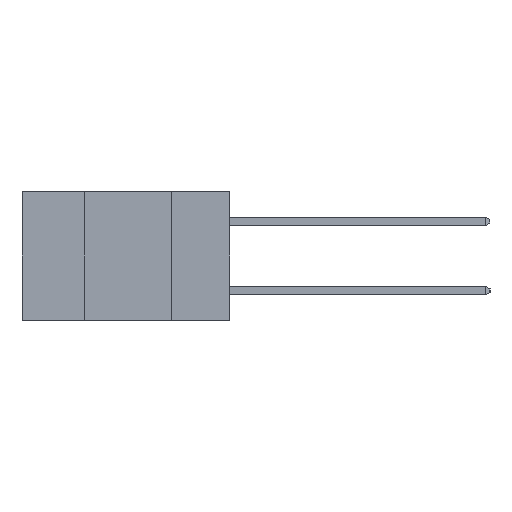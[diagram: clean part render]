
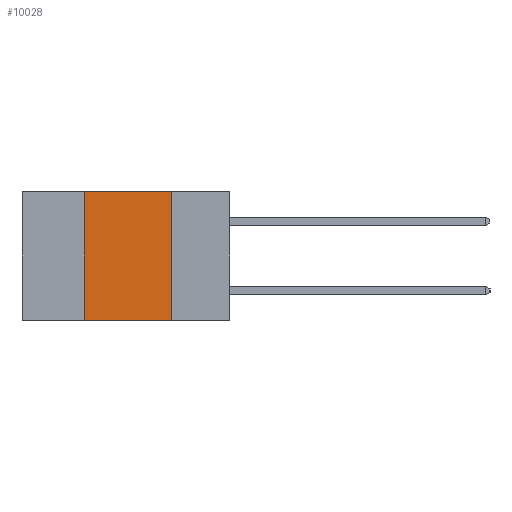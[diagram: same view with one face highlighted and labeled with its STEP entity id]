
A CAD part, left-side view. The second image highlights one B-rep face of the part: STEP entity #10028.
In plain terms, the highlighted planar face has unit normal (-1, 0, 0).
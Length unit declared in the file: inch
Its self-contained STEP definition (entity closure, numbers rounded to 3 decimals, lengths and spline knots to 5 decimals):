
#29 = DIRECTION ( 'NONE',  ( 0., 0., 1. ) ) ;
#115 = LINE ( 'NONE', #14976, #8903 ) ;
#502 = CARTESIAN_POINT ( 'NONE',  ( 0., 0.17, -0.37 ) ) ;
#624 = ORIENTED_EDGE ( 'NONE', *, *, #6920, .T. ) ;
#657 = CARTESIAN_POINT ( 'NONE',  ( 0., 0.42, 0. ) ) ;
#780 = VERTEX_POINT ( 'NONE', #4286 ) ;
#1017 = EDGE_CURVE ( 'NONE', #4652, #780, #13399, .T. ) ;
#2621 = ORIENTED_EDGE ( 'NONE', *, *, #6716, .F. ) ;
#3470 = AXIS2_PLACEMENT_3D ( 'NONE', #11093, #11650, #11632 ) ;
#3851 = EDGE_LOOP ( 'NONE', ( #14650, #2621, #12785, #624 ) ) ;
#4035 = VECTOR ( 'NONE', #13903, 39.37008 ) ;
#4286 = CARTESIAN_POINT ( 'NONE',  ( 0., 0.17, -0.37 ) ) ;
#4652 = VERTEX_POINT ( 'NONE', #10994 ) ;
#4947 = FACE_OUTER_BOUND ( 'NONE', #3851, .T. ) ;
#6237 = LINE ( 'NONE', #13095, #14942 ) ;
#6617 = VERTEX_POINT ( 'NONE', #11918 ) ;
#6716 = EDGE_CURVE ( 'NONE', #13070, #4652, #6237, .T. ) ;
#6920 = EDGE_CURVE ( 'NONE', #6617, #780, #12240, .T. ) ;
#6927 = DIRECTION ( 'NONE',  ( 0., -1., 0. ) ) ;
#7450 = CARTESIAN_POINT ( 'NONE',  ( 0., 0.6, -0.37 ) ) ;
#8903 = VECTOR ( 'NONE', #29, 39.37008 ) ;
#9192 = VECTOR ( 'NONE', #6927, 39.37008 ) ;
#10028 = ADVANCED_FACE ( 'NONE', ( #4947 ), #12521, .F. ) ;
#10836 = EDGE_CURVE ( 'NONE', #6617, #13070, #115, .T. ) ;
#10994 = CARTESIAN_POINT ( 'NONE',  ( 0., 0.17, 0. ) ) ;
#11093 = CARTESIAN_POINT ( 'NONE',  ( 0., 0.6, 0. ) ) ;
#11632 = DIRECTION ( 'NONE',  ( 0., 0., -1. ) ) ;
#11650 = DIRECTION ( 'NONE',  ( 1., 0., 0. ) ) ;
#11918 = CARTESIAN_POINT ( 'NONE',  ( 0., 0.42, -0.37 ) ) ;
#12240 = LINE ( 'NONE', #7450, #9192 ) ;
#12372 = DIRECTION ( 'NONE',  ( 0., -1., 0. ) ) ;
#12521 = PLANE ( 'NONE',  #3470 ) ;
#12785 = ORIENTED_EDGE ( 'NONE', *, *, #10836, .F. ) ;
#13070 = VERTEX_POINT ( 'NONE', #657 ) ;
#13095 = CARTESIAN_POINT ( 'NONE',  ( 0., 0.6, 0. ) ) ;
#13399 = LINE ( 'NONE', #502, #4035 ) ;
#13903 = DIRECTION ( 'NONE',  ( 0., 0., -1. ) ) ;
#14650 = ORIENTED_EDGE ( 'NONE', *, *, #1017, .F. ) ;
#14942 = VECTOR ( 'NONE', #12372, 39.37008 ) ;
#14976 = CARTESIAN_POINT ( 'NONE',  ( 0., 0.42, -0.37 ) ) ;
